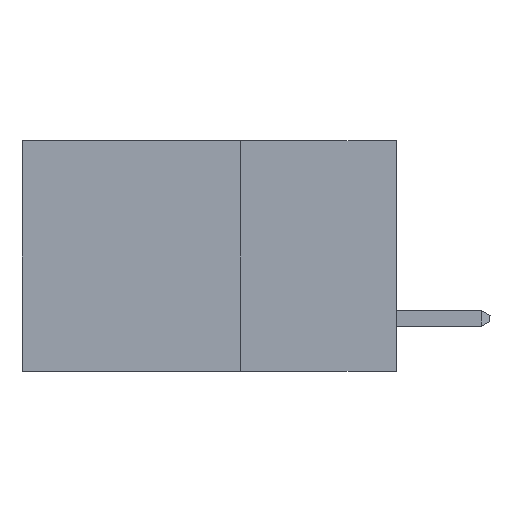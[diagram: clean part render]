
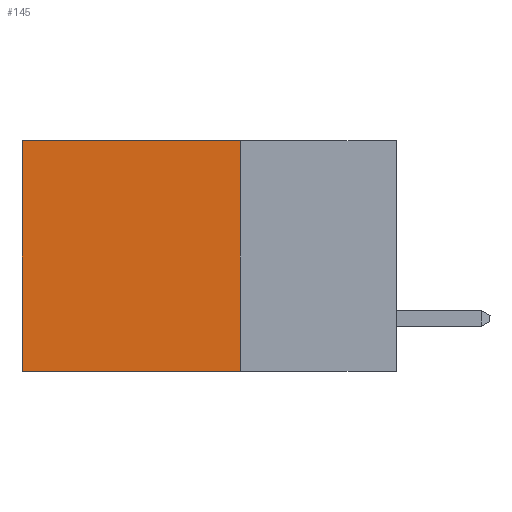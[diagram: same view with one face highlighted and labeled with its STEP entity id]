
A CAD part, left-side view. The second image highlights one B-rep face of the part: STEP entity #145.
In plain terms, the highlighted planar face has unit normal (-1, 0, 0).
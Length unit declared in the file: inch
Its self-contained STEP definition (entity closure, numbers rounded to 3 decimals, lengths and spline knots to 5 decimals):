
#145 = ADVANCED_FACE ( 'NONE', ( #8587 ), #13841, .F. ) ;
#563 = CARTESIAN_POINT ( 'NONE',  ( 0.2615, 0.6, -0.37 ) ) ;
#689 = DIRECTION ( 'NONE',  ( 0., 0., -1. ) ) ;
#1914 = DIRECTION ( 'NONE',  ( 1., 0., 0. ) ) ;
#2266 = ORIENTED_EDGE ( 'NONE', *, *, #13490, .F. ) ;
#2405 = EDGE_CURVE ( 'NONE', #5801, #8253, #13784, .T. ) ;
#2664 = AXIS2_PLACEMENT_3D ( 'NONE', #13993, #1914, #689 ) ;
#2891 = DIRECTION ( 'NONE',  ( 0., 0., -1. ) ) ;
#2907 = DIRECTION ( 'NONE',  ( 0., 1., 0. ) ) ;
#3802 = CARTESIAN_POINT ( 'NONE',  ( 0.2615, 0.25, -0.37 ) ) ;
#3815 = DIRECTION ( 'NONE',  ( 0., 0., -1. ) ) ;
#4014 = EDGE_LOOP ( 'NONE', ( #7566, #2266, #9476, #5347 ) ) ;
#4033 = CARTESIAN_POINT ( 'NONE',  ( 0.2615, 0.25, 0. ) ) ;
#4731 = CARTESIAN_POINT ( 'NONE',  ( 0.2615, 0.6, 0. ) ) ;
#5095 = LINE ( 'NONE', #13974, #11792 ) ;
#5347 = ORIENTED_EDGE ( 'NONE', *, *, #10256, .T. ) ;
#5381 = VERTEX_POINT ( 'NONE', #3802 ) ;
#5398 = VECTOR ( 'NONE', #11998, 39.37008 ) ;
#5562 = CARTESIAN_POINT ( 'NONE',  ( 0.2615, 0.6, -0.37 ) ) ;
#5801 = VERTEX_POINT ( 'NONE', #4731 ) ;
#6890 = VERTEX_POINT ( 'NONE', #4033 ) ;
#7566 = ORIENTED_EDGE ( 'NONE', *, *, #2405, .T. ) ;
#7656 = CARTESIAN_POINT ( 'NONE',  ( 0.2615, 0.25, -0.37 ) ) ;
#8253 = VERTEX_POINT ( 'NONE', #5562 ) ;
#8412 = CARTESIAN_POINT ( 'NONE',  ( 0.2615, 0.25, -0.37 ) ) ;
#8587 = FACE_OUTER_BOUND ( 'NONE', #4014, .T. ) ;
#9476 = ORIENTED_EDGE ( 'NONE', *, *, #11151, .F. ) ;
#9626 = LINE ( 'NONE', #8412, #12997 ) ;
#10256 = EDGE_CURVE ( 'NONE', #6890, #5801, #5095, .T. ) ;
#11132 = VECTOR ( 'NONE', #3815, 39.37008 ) ;
#11151 = EDGE_CURVE ( 'NONE', #6890, #5381, #9626, .T. ) ;
#11792 = VECTOR ( 'NONE', #2907, 39.37008 ) ;
#11998 = DIRECTION ( 'NONE',  ( 0., 1., 0. ) ) ;
#12997 = VECTOR ( 'NONE', #2891, 39.37008 ) ;
#13037 = LINE ( 'NONE', #7656, #5398 ) ;
#13490 = EDGE_CURVE ( 'NONE', #5381, #8253, #13037, .T. ) ;
#13784 = LINE ( 'NONE', #563, #11132 ) ;
#13841 = PLANE ( 'NONE',  #2664 ) ;
#13974 = CARTESIAN_POINT ( 'NONE',  ( 0.2615, 0.25, 0. ) ) ;
#13993 = CARTESIAN_POINT ( 'NONE',  ( 0.2615, 0.25, -0.37 ) ) ;
